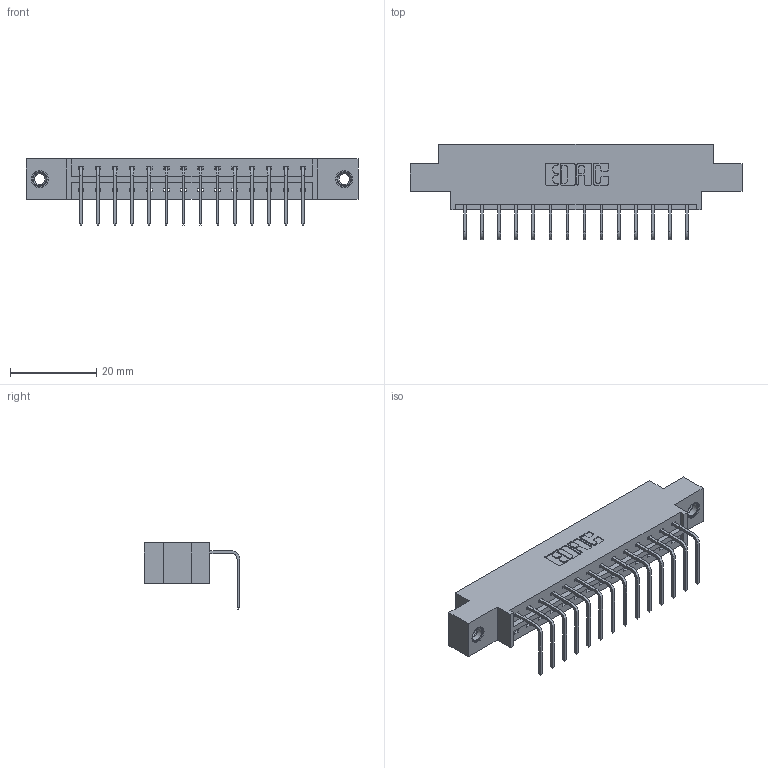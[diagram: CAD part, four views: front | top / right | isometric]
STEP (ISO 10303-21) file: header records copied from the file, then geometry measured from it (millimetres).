
FILE_DESCRIPTION (( 'STEP AP203' ), '1' );
FILE_NAME ('833-014-558-607.STEP', '2020-05-31T14:56:08', ( '' ), ( '' ), 'SwSTEP 2.0', 'SolidWorks 2020', '' );
FILE_SCHEMA (( 'CONFIG_CONTROL_DESIGN' ));
Length unit declared in the file: inch
Products named in the file (4): 345-250-001_345-250-005-103; 833-014-558-607; 833 Part_Offset - .156 Dia - TI; 345-292-001_558 Tail - 2
Assembly tree (17 placements, depth 2):
  833-014-558-607
    833 Part_Offset - .156 Dia - TI
    345-292-001_558 Tail - 2  x14
    345-250-001_345-250-005-103  x2
Bounding box: 77.01 x 22.17 x 15.37 mm (x, y, z)
Volume: 7314.2 mm3; surface area: 8252.1 mm2
Topology: 17 solids, 17 shells, 1018 faces, 3007 edges, 1978 vertices
Faces by surface type: plane 722, cylinder 280, cone 12, torus 4
Entity records: 13582 total; most frequent: CARTESIAN_POINT 2331, ORIENTED_EDGE 2274, DIRECTION 2055, EDGE_CURVE 1137, LINE 989, VECTOR 989, VERTEX_POINT 752, AXIS2_PLACEMENT_3D 533
